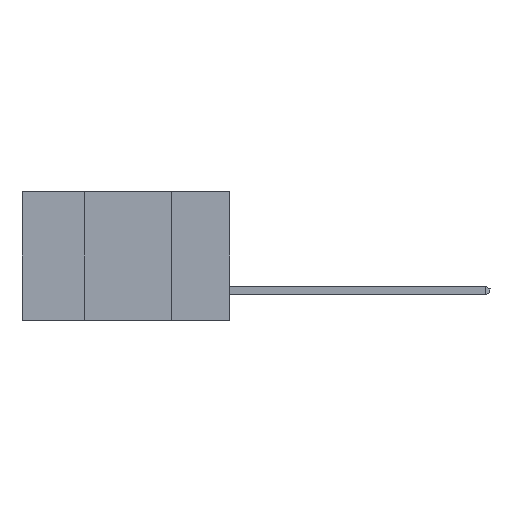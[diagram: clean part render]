
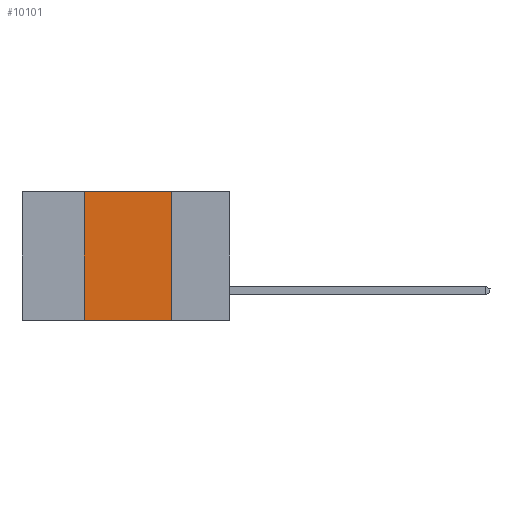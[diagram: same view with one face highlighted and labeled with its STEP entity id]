
A CAD part, left-side view. The second image highlights one B-rep face of the part: STEP entity #10101.
In plain terms, the highlighted planar face has unit normal (-1, 0, 0).
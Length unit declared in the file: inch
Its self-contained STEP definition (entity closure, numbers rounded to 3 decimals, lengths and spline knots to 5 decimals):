
#1044 = CARTESIAN_POINT ( 'NONE',  ( 0., 0.42, -0.37 ) ) ;
#1054 = DIRECTION ( 'NONE',  ( 0., 0., -1. ) ) ;
#1115 = DIRECTION ( 'NONE',  ( 0., 0., 1. ) ) ;
#1143 = EDGE_CURVE ( 'NONE', #15804, #9464, #4062, .T. ) ;
#1227 = ORIENTED_EDGE ( 'NONE', *, *, #10887, .F. ) ;
#2616 = CARTESIAN_POINT ( 'NONE',  ( 0., 0.17, -0.37 ) ) ;
#3141 = CARTESIAN_POINT ( 'NONE',  ( 0., 0.17, 0. ) ) ;
#3598 = LINE ( 'NONE', #18750, #11569 ) ;
#4062 = LINE ( 'NONE', #2616, #8427 ) ;
#4616 = DIRECTION ( 'NONE',  ( 1., 0., 0. ) ) ;
#4684 = AXIS2_PLACEMENT_3D ( 'NONE', #7569, #4616, #6000 ) ;
#6000 = DIRECTION ( 'NONE',  ( 0., 0., -1. ) ) ;
#7402 = CARTESIAN_POINT ( 'NONE',  ( 0., 0.6, -0.37 ) ) ;
#7569 = CARTESIAN_POINT ( 'NONE',  ( 0., 0.6, 0. ) ) ;
#7870 = VECTOR ( 'NONE', #13362, 39.37008 ) ;
#8061 = ORIENTED_EDGE ( 'NONE', *, *, #18032, .T. ) ;
#8399 = ORIENTED_EDGE ( 'NONE', *, *, #1143, .F. ) ;
#8427 = VECTOR ( 'NONE', #1054, 39.37008 ) ;
#8848 = ORIENTED_EDGE ( 'NONE', *, *, #11497, .F. ) ;
#9464 = VERTEX_POINT ( 'NONE', #13072 ) ;
#9579 = DIRECTION ( 'NONE',  ( 0., -1., 0. ) ) ;
#9925 = LINE ( 'NONE', #14800, #17515 ) ;
#10101 = ADVANCED_FACE ( 'NONE', ( #14994 ), #17617, .F. ) ;
#10887 = EDGE_CURVE ( 'NONE', #14438, #15804, #3598, .T. ) ;
#11497 = EDGE_CURVE ( 'NONE', #12953, #14438, #9925, .T. ) ;
#11569 = VECTOR ( 'NONE', #9579, 39.37008 ) ;
#12570 = CARTESIAN_POINT ( 'NONE',  ( 0., 0.42, 0. ) ) ;
#12953 = VERTEX_POINT ( 'NONE', #1044 ) ;
#13072 = CARTESIAN_POINT ( 'NONE',  ( 0., 0.17, -0.37 ) ) ;
#13362 = DIRECTION ( 'NONE',  ( 0., -1., 0. ) ) ;
#14283 = EDGE_LOOP ( 'NONE', ( #8399, #1227, #8848, #8061 ) ) ;
#14438 = VERTEX_POINT ( 'NONE', #12570 ) ;
#14800 = CARTESIAN_POINT ( 'NONE',  ( 0., 0.42, -0.37 ) ) ;
#14994 = FACE_OUTER_BOUND ( 'NONE', #14283, .T. ) ;
#15804 = VERTEX_POINT ( 'NONE', #3141 ) ;
#16569 = LINE ( 'NONE', #7402, #7870 ) ;
#17515 = VECTOR ( 'NONE', #1115, 39.37008 ) ;
#17617 = PLANE ( 'NONE',  #4684 ) ;
#18032 = EDGE_CURVE ( 'NONE', #12953, #9464, #16569, .T. ) ;
#18750 = CARTESIAN_POINT ( 'NONE',  ( 0., 0.6, 0. ) ) ;
